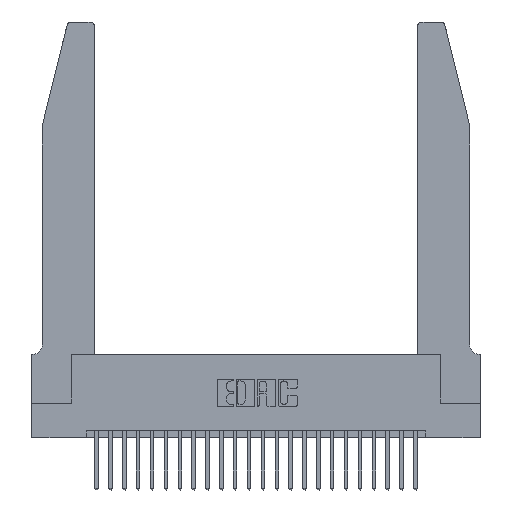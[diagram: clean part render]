
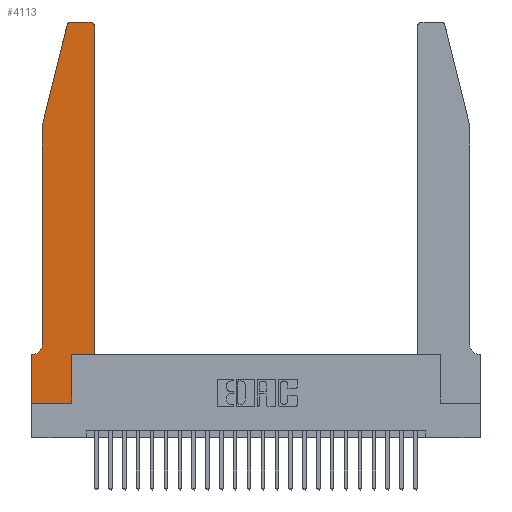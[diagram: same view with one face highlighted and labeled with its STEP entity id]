
A CAD part, top view. The second image highlights one B-rep face of the part: STEP entity #4113.
In plain terms, the highlighted planar face has unit normal (0, 0, 1).
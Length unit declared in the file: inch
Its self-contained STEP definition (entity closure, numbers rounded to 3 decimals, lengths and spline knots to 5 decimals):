
#242 = VERTEX_POINT ( 'NONE', #7997 ) ;
#833 = DIRECTION ( 'NONE',  ( -1., 0., 0. ) ) ;
#996 = VERTEX_POINT ( 'NONE', #6297 ) ;
#1058 = CIRCLE ( 'NONE', #13363, 0.03 ) ;
#1068 = ORIENTED_EDGE ( 'NONE', *, *, #10764, .T. ) ;
#1175 = EDGE_CURVE ( 'NONE', #16499, #22149, #11165, .T. ) ;
#1360 = CARTESIAN_POINT ( 'NONE',  ( 0.284, 2.75, 0.37 ) ) ;
#1364 = PLANE ( 'NONE',  #26011 ) ;
#1567 = VECTOR ( 'NONE', #2433, 39.37008 ) ;
#1856 = LINE ( 'NONE', #24513, #6625 ) ;
#2011 = FACE_OUTER_BOUND ( 'NONE', #12648, .T. ) ;
#2433 = DIRECTION ( 'NONE',  ( -0.239, -0.971, 0. ) ) ;
#2569 = EDGE_CURVE ( 'NONE', #6489, #15345, #10261, .T. ) ;
#3483 = DIRECTION ( 'NONE',  ( 1., 0., 0. ) ) ;
#4013 = DIRECTION ( 'NONE',  ( 0., 0., 1. ) ) ;
#4113 = ADVANCED_FACE ( 'NONE', ( #2011 ), #1364, .T. ) ;
#4630 = EDGE_CURVE ( 'NONE', #19805, #15819, #1058, .T. ) ;
#4737 = ORIENTED_EDGE ( 'NONE', *, *, #4630, .T. ) ;
#5513 = ORIENTED_EDGE ( 'NONE', *, *, #21434, .T. ) ;
#5780 = ORIENTED_EDGE ( 'NONE', *, *, #2569, .T. ) ;
#5893 = CARTESIAN_POINT ( 'NONE',  ( 0.2865, 0.35, 0.37 ) ) ;
#6134 = CARTESIAN_POINT ( 'NONE',  ( 0.4505, 0.35, 0.37 ) ) ;
#6228 = LINE ( 'NONE', #5893, #14369 ) ;
#6297 = CARTESIAN_POINT ( 'NONE',  ( 0.4505, 0.35, 0.37 ) ) ;
#6489 = VERTEX_POINT ( 'NONE', #17370 ) ;
#6625 = VECTOR ( 'NONE', #833, 39.37008 ) ;
#6919 = VERTEX_POINT ( 'NONE', #12406 ) ;
#7054 = DIRECTION ( 'NONE',  ( 0., 1., 0. ) ) ;
#7553 = CARTESIAN_POINT ( 'NONE',  ( 0.25487, 2.72718, 0.37 ) ) ;
#7997 = CARTESIAN_POINT ( 'NONE',  ( 0.2865, 0., 0.37 ) ) ;
#8008 = CIRCLE ( 'NONE', #22977, 0.07 ) ;
#9304 = DIRECTION ( 'NONE',  ( 1., 0., 0. ) ) ;
#9509 = EDGE_CURVE ( 'NONE', #6919, #19805, #21532, .T. ) ;
#9650 = VECTOR ( 'NONE', #12953, 39.37008 ) ;
#9733 = ORIENTED_EDGE ( 'NONE', *, *, #16624, .T. ) ;
#10136 = VERTEX_POINT ( 'NONE', #13977 ) ;
#10222 = DIRECTION ( 'NONE',  ( 0., -1., 0. ) ) ;
#10223 = VERTEX_POINT ( 'NONE', #18482 ) ;
#10261 = LINE ( 'NONE', #18428, #9650 ) ;
#10764 = EDGE_CURVE ( 'NONE', #22149, #242, #17420, .T. ) ;
#11165 = LINE ( 'NONE', #24383, #24715 ) ;
#11550 = ORIENTED_EDGE ( 'NONE', *, *, #18671, .T. ) ;
#11626 = CARTESIAN_POINT ( 'NONE',  ( 0., 0., 0.37 ) ) ;
#11628 = CARTESIAN_POINT ( 'NONE',  ( 0.2605, 2.75, 0.37 ) ) ;
#11691 = DIRECTION ( 'NONE',  ( 1., 0., 0. ) ) ;
#11774 = AXIS2_PLACEMENT_3D ( 'NONE', #17770, #13706, #11691 ) ;
#12406 = CARTESIAN_POINT ( 'NONE',  ( 0.4205, 2.75, 0.37 ) ) ;
#12538 = VECTOR ( 'NONE', #20020, 39.37008 ) ;
#12648 = EDGE_LOOP ( 'NONE', ( #18016, #4737, #11550, #5780, #9733, #16203, #13257, #1068, #21398, #5513, #22824, #24691 ) ) ;
#12707 = CARTESIAN_POINT ( 'NONE',  ( 0.0755, 0.42, 0.37 ) ) ;
#12953 = DIRECTION ( 'NONE',  ( 0., -1., 0. ) ) ;
#13257 = ORIENTED_EDGE ( 'NONE', *, *, #1175, .T. ) ;
#13334 = VECTOR ( 'NONE', #13631, 39.37008 ) ;
#13363 = AXIS2_PLACEMENT_3D ( 'NONE', #24072, #4013, #25894 ) ;
#13631 = DIRECTION ( 'NONE',  ( -1., 0., 0. ) ) ;
#13706 = DIRECTION ( 'NONE',  ( 0., 0., 1. ) ) ;
#13977 = CARTESIAN_POINT ( 'NONE',  ( 0.2865, 0.35, 0.37 ) ) ;
#14369 = VECTOR ( 'NONE', #7054, 39.37008 ) ;
#15154 = DIRECTION ( 'NONE',  ( 0., 0., 1. ) ) ;
#15291 = DIRECTION ( 'NONE',  ( 0., 0., -1. ) ) ;
#15345 = VERTEX_POINT ( 'NONE', #12707 ) ;
#15416 = DIRECTION ( 'NONE',  ( 1., 0., 0. ) ) ;
#15458 = CARTESIAN_POINT ( 'NONE',  ( 0.0055, 0.42, 0.37 ) ) ;
#15819 = VERTEX_POINT ( 'NONE', #7553 ) ;
#15930 = CARTESIAN_POINT ( 'NONE',  ( 0.0055, 0.35, 0.37 ) ) ;
#16203 = ORIENTED_EDGE ( 'NONE', *, *, #23626, .T. ) ;
#16499 = VERTEX_POINT ( 'NONE', #18241 ) ;
#16624 = EDGE_CURVE ( 'NONE', #15345, #22176, #8008, .T. ) ;
#16671 = LINE ( 'NONE', #24433, #1567 ) ;
#17370 = CARTESIAN_POINT ( 'NONE',  ( 0.0755, 2., 0.37 ) ) ;
#17420 = LINE ( 'NONE', #11626, #22159 ) ;
#17770 = CARTESIAN_POINT ( 'NONE',  ( 0.4205, 2.72, 0.37 ) ) ;
#18016 = ORIENTED_EDGE ( 'NONE', *, *, #9509, .T. ) ;
#18241 = CARTESIAN_POINT ( 'NONE',  ( 0., 0.35, 0.37 ) ) ;
#18428 = CARTESIAN_POINT ( 'NONE',  ( 0.0755, 2., 0.37 ) ) ;
#18482 = CARTESIAN_POINT ( 'NONE',  ( 0.4505, 2.72, 0.37 ) ) ;
#18671 = EDGE_CURVE ( 'NONE', #15819, #6489, #16671, .T. ) ;
#19203 = CIRCLE ( 'NONE', #11774, 0.03 ) ;
#19373 = EDGE_CURVE ( 'NONE', #996, #10223, #22313, .T. ) ;
#19408 = VECTOR ( 'NONE', #9304, 39.37008 ) ;
#19805 = VERTEX_POINT ( 'NONE', #1360 ) ;
#20020 = DIRECTION ( 'NONE',  ( 0., 1., 0. ) ) ;
#21028 = EDGE_CURVE ( 'NONE', #242, #10136, #6228, .T. ) ;
#21077 = CARTESIAN_POINT ( 'NONE',  ( 0.4505, 0.35, 0.37 ) ) ;
#21398 = ORIENTED_EDGE ( 'NONE', *, *, #21028, .T. ) ;
#21434 = EDGE_CURVE ( 'NONE', #10136, #996, #23537, .T. ) ;
#21532 = LINE ( 'NONE', #11628, #13334 ) ;
#22149 = VERTEX_POINT ( 'NONE', #24069 ) ;
#22159 = VECTOR ( 'NONE', #3483, 39.37008 ) ;
#22176 = VERTEX_POINT ( 'NONE', #15930 ) ;
#22313 = LINE ( 'NONE', #6134, #12538 ) ;
#22824 = ORIENTED_EDGE ( 'NONE', *, *, #19373, .T. ) ;
#22977 = AXIS2_PLACEMENT_3D ( 'NONE', #15458, #15291, #23602 ) ;
#23537 = LINE ( 'NONE', #21077, #19408 ) ;
#23558 = CARTESIAN_POINT ( 'NONE',  ( 0., 0.35, 0.37 ) ) ;
#23602 = DIRECTION ( 'NONE',  ( -1., 0., 0. ) ) ;
#23626 = EDGE_CURVE ( 'NONE', #22176, #16499, #1856, .T. ) ;
#24069 = CARTESIAN_POINT ( 'NONE',  ( 0., 0., 0.37 ) ) ;
#24072 = CARTESIAN_POINT ( 'NONE',  ( 0.284, 2.72, 0.37 ) ) ;
#24383 = CARTESIAN_POINT ( 'NONE',  ( 0., 0., 0.37 ) ) ;
#24433 = CARTESIAN_POINT ( 'NONE',  ( 0.0755, 2., 0.37 ) ) ;
#24513 = CARTESIAN_POINT ( 'NONE',  ( 0.0755, 0.35, 0.37 ) ) ;
#24565 = EDGE_CURVE ( 'NONE', #10223, #6919, #19203, .T. ) ;
#24691 = ORIENTED_EDGE ( 'NONE', *, *, #24565, .T. ) ;
#24715 = VECTOR ( 'NONE', #10222, 39.37008 ) ;
#25894 = DIRECTION ( 'NONE',  ( 1., 0., 0. ) ) ;
#26011 = AXIS2_PLACEMENT_3D ( 'NONE', #23558, #15154, #15416 ) ;
